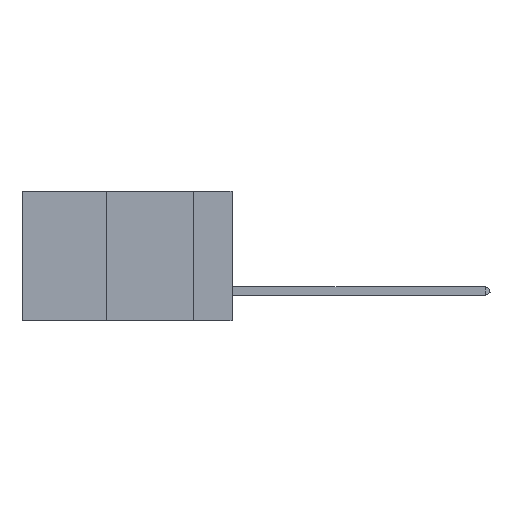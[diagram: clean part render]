
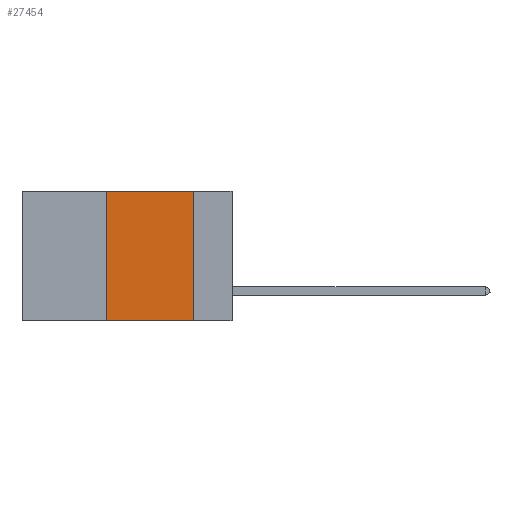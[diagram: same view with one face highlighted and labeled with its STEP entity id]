
A CAD part, left-side view. The second image highlights one B-rep face of the part: STEP entity #27454.
In plain terms, the highlighted planar face has unit normal (-1, 0, 0).
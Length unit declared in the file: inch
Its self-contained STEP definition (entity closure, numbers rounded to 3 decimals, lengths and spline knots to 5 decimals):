
#804 = CARTESIAN_POINT ( 'NONE',  ( 0., 0.36, 0. ) ) ;
#1086 = CARTESIAN_POINT ( 'NONE',  ( 0., 0.36, -0.37 ) ) ;
#1797 = ORIENTED_EDGE ( 'NONE', *, *, #24552, .F. ) ;
#2235 = CARTESIAN_POINT ( 'NONE',  ( 0., 0.36, 0. ) ) ;
#2260 = EDGE_CURVE ( 'NONE', #21135, #36038, #30007, .T. ) ;
#7037 = DIRECTION ( 'NONE',  ( 1., 0., 0. ) ) ;
#7040 = VECTOR ( 'NONE', #23849, 39.37008 ) ;
#8352 = VERTEX_POINT ( 'NONE', #1086 ) ;
#9138 = VECTOR ( 'NONE', #18037, 39.37008 ) ;
#9419 = VECTOR ( 'NONE', #18318, 39.37008 ) ;
#9449 = CARTESIAN_POINT ( 'NONE',  ( 0., 0.11, 0. ) ) ;
#11176 = DIRECTION ( 'NONE',  ( 0., -1., 0. ) ) ;
#13675 = CARTESIAN_POINT ( 'NONE',  ( 0., 0.11, 0. ) ) ;
#13824 = EDGE_LOOP ( 'NONE', ( #35127, #22133, #1797, #36726 ) ) ;
#14397 = AXIS2_PLACEMENT_3D ( 'NONE', #18908, #7037, #15807 ) ;
#15807 = DIRECTION ( 'NONE',  ( 0., 0., -1. ) ) ;
#16052 = VECTOR ( 'NONE', #11176, 39.37008 ) ;
#17207 = LINE ( 'NONE', #32353, #9138 ) ;
#17376 = LINE ( 'NONE', #22453, #16052 ) ;
#17397 = EDGE_CURVE ( 'NONE', #8352, #36038, #17376, .T. ) ;
#18037 = DIRECTION ( 'NONE',  ( 0., -1., 0. ) ) ;
#18318 = DIRECTION ( 'NONE',  ( 0., 0., -1. ) ) ;
#18908 = CARTESIAN_POINT ( 'NONE',  ( 0., 0.6, 0. ) ) ;
#18969 = EDGE_CURVE ( 'NONE', #23684, #21135, #17207, .T. ) ;
#21135 = VERTEX_POINT ( 'NONE', #9449 ) ;
#21164 = CARTESIAN_POINT ( 'NONE',  ( 0., 0.11, -0.37 ) ) ;
#22133 = ORIENTED_EDGE ( 'NONE', *, *, #18969, .F. ) ;
#22453 = CARTESIAN_POINT ( 'NONE',  ( 0., 0.6, -0.37 ) ) ;
#23684 = VERTEX_POINT ( 'NONE', #2235 ) ;
#23849 = DIRECTION ( 'NONE',  ( 0., 0., 1. ) ) ;
#24552 = EDGE_CURVE ( 'NONE', #8352, #23684, #33964, .T. ) ;
#25677 = FACE_OUTER_BOUND ( 'NONE', #13824, .T. ) ;
#27454 = ADVANCED_FACE ( 'NONE', ( #25677 ), #36092, .F. ) ;
#30007 = LINE ( 'NONE', #13675, #9419 ) ;
#32353 = CARTESIAN_POINT ( 'NONE',  ( 0., 0.6, 0. ) ) ;
#33964 = LINE ( 'NONE', #804, #7040 ) ;
#35127 = ORIENTED_EDGE ( 'NONE', *, *, #2260, .F. ) ;
#36038 = VERTEX_POINT ( 'NONE', #21164 ) ;
#36092 = PLANE ( 'NONE',  #14397 ) ;
#36726 = ORIENTED_EDGE ( 'NONE', *, *, #17397, .T. ) ;
